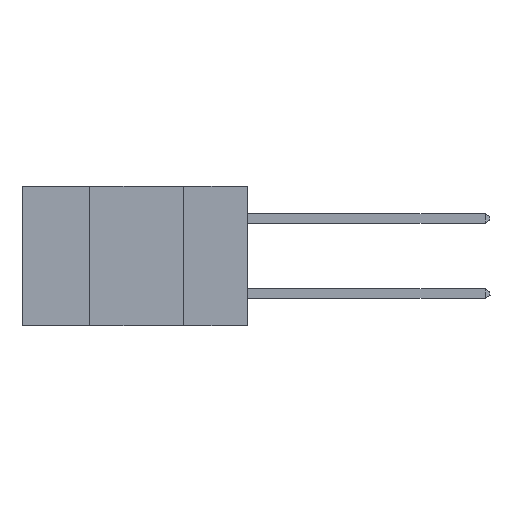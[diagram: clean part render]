
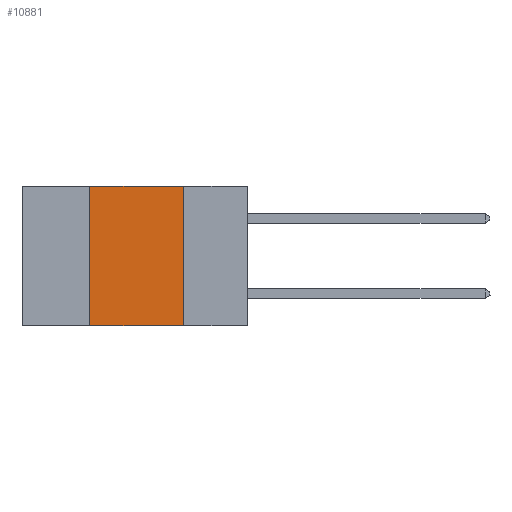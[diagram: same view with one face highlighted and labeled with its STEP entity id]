
A CAD part, left-side view. The second image highlights one B-rep face of the part: STEP entity #10881.
In plain terms, the highlighted planar face has unit normal (-1, 0, 0).
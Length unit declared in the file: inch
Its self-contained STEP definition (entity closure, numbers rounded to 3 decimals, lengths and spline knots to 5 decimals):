
#83 = DIRECTION ( 'NONE',  ( 0., 0., 1. ) ) ;
#266 = CARTESIAN_POINT ( 'NONE',  ( 0., 0.42, 0. ) ) ;
#322 = CARTESIAN_POINT ( 'NONE',  ( 0., 0.42, -0.37 ) ) ;
#381 = LINE ( 'NONE', #4479, #4700 ) ;
#515 = VECTOR ( 'NONE', #83, 39.37008 ) ;
#673 = EDGE_CURVE ( 'NONE', #7547, #3973, #381, .T. ) ;
#1462 = VERTEX_POINT ( 'NONE', #266 ) ;
#1549 = CARTESIAN_POINT ( 'NONE',  ( 0., 0.17, 0. ) ) ;
#1687 = AXIS2_PLACEMENT_3D ( 'NONE', #6021, #4430, #2516 ) ;
#1899 = FACE_OUTER_BOUND ( 'NONE', #9667, .T. ) ;
#2032 = ORIENTED_EDGE ( 'NONE', *, *, #673, .F. ) ;
#2516 = DIRECTION ( 'NONE',  ( 0., 0., -1. ) ) ;
#3006 = LINE ( 'NONE', #7915, #3832 ) ;
#3810 = DIRECTION ( 'NONE',  ( 0., 0., -1. ) ) ;
#3832 = VECTOR ( 'NONE', #5192, 39.37008 ) ;
#3964 = CARTESIAN_POINT ( 'NONE',  ( 0., 0.17, -0.37 ) ) ;
#3973 = VERTEX_POINT ( 'NONE', #3964 ) ;
#4430 = DIRECTION ( 'NONE',  ( 1., 0., 0. ) ) ;
#4479 = CARTESIAN_POINT ( 'NONE',  ( 0., 0.17, 0. ) ) ;
#4576 = VECTOR ( 'NONE', #8946, 39.37008 ) ;
#4700 = VECTOR ( 'NONE', #3810, 39.37008 ) ;
#5174 = ORIENTED_EDGE ( 'NONE', *, *, #10387, .F. ) ;
#5192 = DIRECTION ( 'NONE',  ( 0., -1., 0. ) ) ;
#5314 = ORIENTED_EDGE ( 'NONE', *, *, #10919, .F. ) ;
#5564 = CARTESIAN_POINT ( 'NONE',  ( 0., 0.6, -0.37 ) ) ;
#6021 = CARTESIAN_POINT ( 'NONE',  ( 0., 0.6, 0. ) ) ;
#7547 = VERTEX_POINT ( 'NONE', #1549 ) ;
#7572 = ORIENTED_EDGE ( 'NONE', *, *, #10502, .T. ) ;
#7915 = CARTESIAN_POINT ( 'NONE',  ( 0., 0.6, 0. ) ) ;
#8946 = DIRECTION ( 'NONE',  ( 0., -1., 0. ) ) ;
#9202 = LINE ( 'NONE', #5564, #4576 ) ;
#9566 = CARTESIAN_POINT ( 'NONE',  ( 0., 0.42, 0. ) ) ;
#9667 = EDGE_LOOP ( 'NONE', ( #2032, #5174, #5314, #7572 ) ) ;
#10387 = EDGE_CURVE ( 'NONE', #1462, #7547, #3006, .T. ) ;
#10458 = VERTEX_POINT ( 'NONE', #322 ) ;
#10502 = EDGE_CURVE ( 'NONE', #10458, #3973, #9202, .T. ) ;
#10881 = ADVANCED_FACE ( 'NONE', ( #1899 ), #11369, .F. ) ;
#10919 = EDGE_CURVE ( 'NONE', #10458, #1462, #10968, .T. ) ;
#10968 = LINE ( 'NONE', #9566, #515 ) ;
#11369 = PLANE ( 'NONE',  #1687 ) ;
